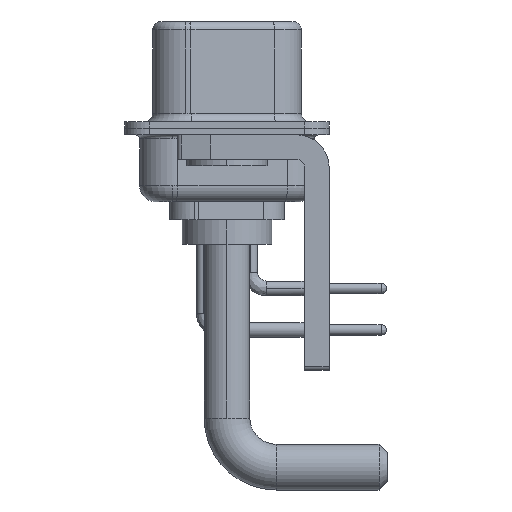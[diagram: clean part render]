
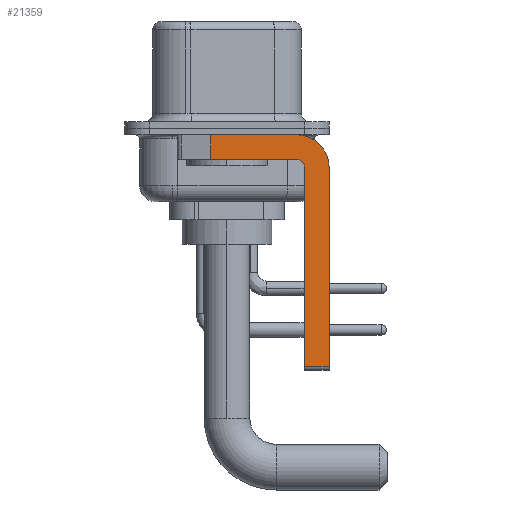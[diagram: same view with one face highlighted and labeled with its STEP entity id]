
A CAD part, left-side view. The second image highlights one B-rep face of the part: STEP entity #21359.
In plain terms, the highlighted planar face has unit normal (-1, 0, 0).
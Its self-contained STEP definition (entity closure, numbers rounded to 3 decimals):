
#396 = CIRCLE ( 'NONE', #2252, 0.5 ) ;
#765 = CIRCLE ( 'NONE', #5407, 2. ) ;
#971 = CARTESIAN_POINT ( 'NONE',  ( -2.9, -4.25, -1.9 ) ) ;
#1142 = CARTESIAN_POINT ( 'NONE',  ( -2.9, -4.25, -2.4 ) ) ;
#1424 = DIRECTION ( 'NONE',  ( 1., 0., 0. ) ) ;
#1478 = LINE ( 'NONE', #26280, #19015 ) ;
#1630 = DIRECTION ( 'NONE',  ( 0., -1., 0. ) ) ;
#1825 = VERTEX_POINT ( 'NONE', #21537 ) ;
#1877 = CARTESIAN_POINT ( 'NONE',  ( -2.9, 0.978, -0.4 ) ) ;
#1933 = ORIENTED_EDGE ( 'NONE', *, *, #19990, .F. ) ;
#2252 = AXIS2_PLACEMENT_3D ( 'NONE', #8468, #6315, #4570 ) ;
#2510 = LINE ( 'NONE', #2651, #11771 ) ;
#2558 = DIRECTION ( 'NONE',  ( 0., 1., 0. ) ) ;
#2651 = CARTESIAN_POINT ( 'NONE',  ( -2.9, -4.75, -14.8 ) ) ;
#2924 = EDGE_CURVE ( 'NONE', #1825, #23024, #765, .T. ) ;
#2948 = CARTESIAN_POINT ( 'NONE',  ( -2.9, -4.25, -1.9 ) ) ;
#3130 = LINE ( 'NONE', #971, #3893 ) ;
#3893 = VECTOR ( 'NONE', #2558, 1000. ) ;
#4570 = DIRECTION ( 'NONE',  ( 0., 0., 1. ) ) ;
#5034 = CARTESIAN_POINT ( 'NONE',  ( -2.9, -4.75, -14.55 ) ) ;
#5303 = VECTOR ( 'NONE', #9512, 1000. ) ;
#5407 = AXIS2_PLACEMENT_3D ( 'NONE', #21092, #23425, #18479 ) ;
#6315 = DIRECTION ( 'NONE',  ( -1., 0., 0. ) ) ;
#6401 = EDGE_CURVE ( 'NONE', #20080, #15196, #3130, .T. ) ;
#7018 = LINE ( 'NONE', #24453, #7971 ) ;
#7186 = LINE ( 'NONE', #22845, #18648 ) ;
#7971 = VECTOR ( 'NONE', #13701, 1000. ) ;
#8024 = EDGE_CURVE ( 'NONE', #27269, #21830, #2510, .T. ) ;
#8468 = CARTESIAN_POINT ( 'NONE',  ( -2.9, -4.25, -2.4 ) ) ;
#8823 = CARTESIAN_POINT ( 'NONE',  ( -2.9, -6.25, -14.55 ) ) ;
#9512 = DIRECTION ( 'NONE',  ( 0., -1., 0. ) ) ;
#10383 = EDGE_LOOP ( 'NONE', ( #24618, #13574, #17728, #1933, #18679, #19196, #11346, #23147 ) ) ;
#11346 = ORIENTED_EDGE ( 'NONE', *, *, #27231, .F. ) ;
#11771 = VECTOR ( 'NONE', #26879, 1000. ) ;
#12469 = CARTESIAN_POINT ( 'NONE',  ( -2.9, -4.75, -2.4 ) ) ;
#13574 = ORIENTED_EDGE ( 'NONE', *, *, #25544, .T. ) ;
#13701 = DIRECTION ( 'NONE',  ( 0., 0., -1. ) ) ;
#14026 = EDGE_CURVE ( 'NONE', #27269, #21972, #1478, .T. ) ;
#14888 = FACE_OUTER_BOUND ( 'NONE', #10383, .T. ) ;
#15196 = VERTEX_POINT ( 'NONE', #18150 ) ;
#15954 = VERTEX_POINT ( 'NONE', #1877 ) ;
#17069 = DIRECTION ( 'NONE',  ( 0., 0., -1. ) ) ;
#17728 = ORIENTED_EDGE ( 'NONE', *, *, #6401, .F. ) ;
#18150 = CARTESIAN_POINT ( 'NONE',  ( -2.9, 0.978, -1.9 ) ) ;
#18479 = DIRECTION ( 'NONE',  ( 0., 0., -1. ) ) ;
#18481 = LINE ( 'NONE', #27352, #5303 ) ;
#18648 = VECTOR ( 'NONE', #25178, 1000. ) ;
#18679 = ORIENTED_EDGE ( 'NONE', *, *, #8024, .F. ) ;
#19015 = VECTOR ( 'NONE', #1630, 1000. ) ;
#19196 = ORIENTED_EDGE ( 'NONE', *, *, #14026, .T. ) ;
#19990 = EDGE_CURVE ( 'NONE', #21830, #20080, #396, .T. ) ;
#20080 = VERTEX_POINT ( 'NONE', #2948 ) ;
#20492 = CARTESIAN_POINT ( 'NONE',  ( -2.9, -6.25, -2.4 ) ) ;
#21092 = CARTESIAN_POINT ( 'NONE',  ( -2.9, -4.25, -2.4 ) ) ;
#21359 = ADVANCED_FACE ( 'NONE', ( #14888 ), #23592, .F. ) ;
#21537 = CARTESIAN_POINT ( 'NONE',  ( -2.9, -4.25, -0.4 ) ) ;
#21830 = VERTEX_POINT ( 'NONE', #12469 ) ;
#21972 = VERTEX_POINT ( 'NONE', #8823 ) ;
#22679 = AXIS2_PLACEMENT_3D ( 'NONE', #1142, #1424, #17069 ) ;
#22845 = CARTESIAN_POINT ( 'NONE',  ( -2.9, -6.25, -2.4 ) ) ;
#23024 = VERTEX_POINT ( 'NONE', #20492 ) ;
#23147 = ORIENTED_EDGE ( 'NONE', *, *, #2924, .F. ) ;
#23425 = DIRECTION ( 'NONE',  ( 1., 0., 0. ) ) ;
#23592 = PLANE ( 'NONE',  #22679 ) ;
#24453 = CARTESIAN_POINT ( 'NONE',  ( -2.9, 0.978, -1.9 ) ) ;
#24618 = ORIENTED_EDGE ( 'NONE', *, *, #28584, .F. ) ;
#25178 = DIRECTION ( 'NONE',  ( 0., 0., -1. ) ) ;
#25544 = EDGE_CURVE ( 'NONE', #15954, #15196, #7018, .T. ) ;
#26280 = CARTESIAN_POINT ( 'NONE',  ( -2.9, -4.25, -14.55 ) ) ;
#26879 = DIRECTION ( 'NONE',  ( 0., 0., 1. ) ) ;
#27231 = EDGE_CURVE ( 'NONE', #23024, #21972, #7186, .T. ) ;
#27269 = VERTEX_POINT ( 'NONE', #5034 ) ;
#27352 = CARTESIAN_POINT ( 'NONE',  ( -2.9, 3., -0.4 ) ) ;
#28584 = EDGE_CURVE ( 'NONE', #15954, #1825, #18481, .T. ) ;
